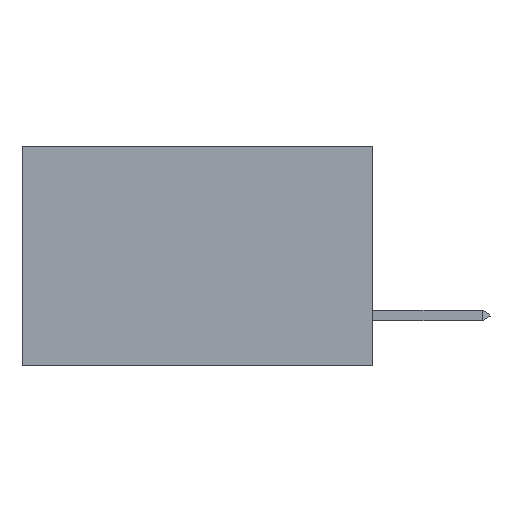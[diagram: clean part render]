
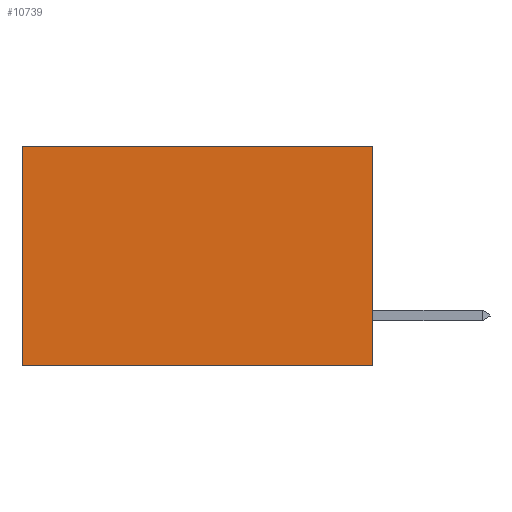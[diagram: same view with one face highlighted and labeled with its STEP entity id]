
A CAD part, left-side view. The second image highlights one B-rep face of the part: STEP entity #10739.
In plain terms, the highlighted planar face has unit normal (-1, 0, 0).
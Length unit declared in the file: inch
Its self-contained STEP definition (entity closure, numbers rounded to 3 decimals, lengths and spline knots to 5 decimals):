
#183 = LINE ( 'NONE', #8102, #3126 ) ;
#211 = CARTESIAN_POINT ( 'NONE',  ( 0.277, 0., -0.37 ) ) ;
#989 = DIRECTION ( 'NONE',  ( 0., 0., -1. ) ) ;
#1992 = ORIENTED_EDGE ( 'NONE', *, *, #9067, .F. ) ;
#2203 = CARTESIAN_POINT ( 'NONE',  ( 0.277, 0.59, 0. ) ) ;
#2866 = EDGE_CURVE ( 'NONE', #14807, #9647, #183, .T. ) ;
#3126 = VECTOR ( 'NONE', #7177, 39.37008 ) ;
#3659 = CARTESIAN_POINT ( 'NONE',  ( 0.277, 0., 0. ) ) ;
#4205 = EDGE_CURVE ( 'NONE', #10153, #12073, #15905, .T. ) ;
#4297 = VECTOR ( 'NONE', #989, 39.37008 ) ;
#4573 = DIRECTION ( 'NONE',  ( 0., 0., -1. ) ) ;
#4630 = CARTESIAN_POINT ( 'NONE',  ( 0.277, 0., -0.37 ) ) ;
#4650 = DIRECTION ( 'NONE',  ( 0., 1., 0. ) ) ;
#5263 = PLANE ( 'NONE',  #11387 ) ;
#5507 = ORIENTED_EDGE ( 'NONE', *, *, #2866, .T. ) ;
#5895 = CARTESIAN_POINT ( 'NONE',  ( 0.277, 0.59, -0.37 ) ) ;
#6165 = CARTESIAN_POINT ( 'NONE',  ( 0.277, 0.59, -0.37 ) ) ;
#6481 = DIRECTION ( 'NONE',  ( 0., 0., -1. ) ) ;
#6845 = LINE ( 'NONE', #10833, #7246 ) ;
#7177 = DIRECTION ( 'NONE',  ( 0., 1., 0. ) ) ;
#7246 = VECTOR ( 'NONE', #4573, 39.37008 ) ;
#7601 = LINE ( 'NONE', #5895, #4297 ) ;
#8102 = CARTESIAN_POINT ( 'NONE',  ( 0.277, 0., 0. ) ) ;
#8720 = ORIENTED_EDGE ( 'NONE', *, *, #10390, .T. ) ;
#8733 = FACE_OUTER_BOUND ( 'NONE', #11415, .T. ) ;
#9067 = EDGE_CURVE ( 'NONE', #14807, #10153, #6845, .T. ) ;
#9565 = VECTOR ( 'NONE', #4650, 39.37008 ) ;
#9647 = VERTEX_POINT ( 'NONE', #2203 ) ;
#10153 = VERTEX_POINT ( 'NONE', #11823 ) ;
#10390 = EDGE_CURVE ( 'NONE', #9647, #12073, #7601, .T. ) ;
#10739 = ADVANCED_FACE ( 'NONE', ( #8733 ), #5263, .F. ) ;
#10833 = CARTESIAN_POINT ( 'NONE',  ( 0.277, 0., -0.37 ) ) ;
#11387 = AXIS2_PLACEMENT_3D ( 'NONE', #211, #14067, #6481 ) ;
#11415 = EDGE_LOOP ( 'NONE', ( #8720, #12310, #1992, #5507 ) ) ;
#11823 = CARTESIAN_POINT ( 'NONE',  ( 0.277, 0., -0.37 ) ) ;
#12073 = VERTEX_POINT ( 'NONE', #6165 ) ;
#12310 = ORIENTED_EDGE ( 'NONE', *, *, #4205, .F. ) ;
#14067 = DIRECTION ( 'NONE',  ( 1., 0., 0. ) ) ;
#14807 = VERTEX_POINT ( 'NONE', #3659 ) ;
#15905 = LINE ( 'NONE', #4630, #9565 ) ;
